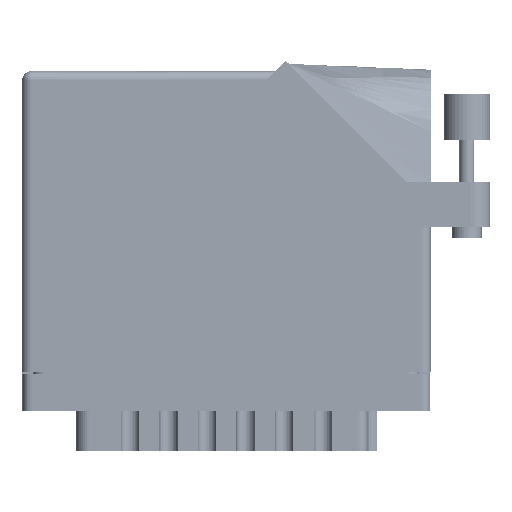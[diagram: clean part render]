
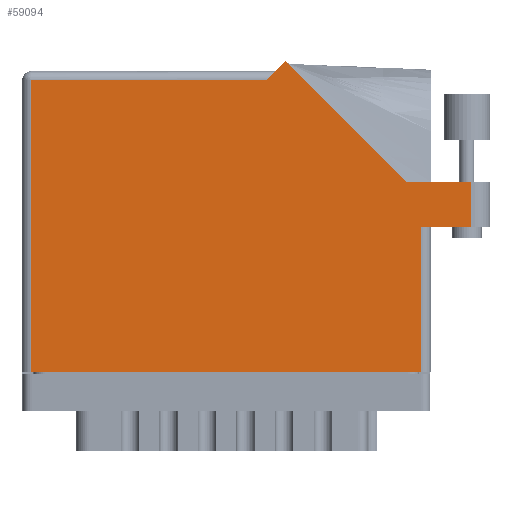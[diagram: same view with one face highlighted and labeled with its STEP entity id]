
A CAD part, front view. The second image highlights one B-rep face of the part: STEP entity #59094.
In plain terms, the highlighted face is planar.
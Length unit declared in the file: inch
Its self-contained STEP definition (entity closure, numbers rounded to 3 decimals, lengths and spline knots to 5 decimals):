
#2067 = ORIENTED_EDGE ( 'NONE', *, *, #8917, .T. ) ;
#4384 = LINE ( 'NONE', #84278, #96605 ) ;
#5635 = DIRECTION ( 'NONE',  ( 0., 0., -1. ) ) ;
#8917 = EDGE_CURVE ( 'NONE', #19180, #78501, #88058, .T. ) ;
#9292 = CARTESIAN_POINT ( 'NONE',  ( 0.062, 0., 0. ) ) ;
#9318 = DIRECTION ( 'NONE',  ( 0., 1., 0. ) ) ;
#10745 = CARTESIAN_POINT ( 'NONE',  ( 3.155, 1.287, 0. ) ) ;
#13589 = CARTESIAN_POINT ( 'NONE',  ( 1.643, 1.968, 0. ) ) ;
#14631 = EDGE_CURVE ( 'NONE', #51018, #41355, #78565, .T. ) ;
#19180 = VERTEX_POINT ( 'NONE', #47078 ) ;
#20090 = ORIENTED_EDGE ( 'NONE', *, *, #83629, .T. ) ;
#20225 = DIRECTION ( 'NONE',  ( -0.707, 0.707, 0. ) ) ;
#20840 = CARTESIAN_POINT ( 'NONE',  ( 2.58942, 1.287, 0. ) ) ;
#21300 = DIRECTION ( 'NONE',  ( -1., 0., 0. ) ) ;
#23514 = VECTOR ( 'NONE', #9318, 39.37008 ) ;
#31052 = EDGE_LOOP ( 'NONE', ( #64737, #20090, #2067, #32978, #32845, #91973, #91093, #93390, #40410 ) ) ;
#31656 = VERTEX_POINT ( 'NONE', #75558 ) ;
#32352 = VECTOR ( 'NONE', #45770, 39.37008 ) ;
#32845 = ORIENTED_EDGE ( 'NONE', *, *, #62433, .T. ) ;
#32978 = ORIENTED_EDGE ( 'NONE', *, *, #67503, .T. ) ;
#32984 = CARTESIAN_POINT ( 'NONE',  ( 1.77571, 2.10071, 0. ) ) ;
#33135 = VECTOR ( 'NONE', #64858, 39.37008 ) ;
#34730 = CARTESIAN_POINT ( 'NONE',  ( 0., 0., 0. ) ) ;
#35352 = CARTESIAN_POINT ( 'NONE',  ( 0., 2.03, 0. ) ) ;
#39279 = DIRECTION ( 'NONE',  ( -0.707, -0.707, 0. ) ) ;
#40410 = ORIENTED_EDGE ( 'NONE', *, *, #59574, .T. ) ;
#41355 = VERTEX_POINT ( 'NONE', #47971 ) ;
#43520 = VECTOR ( 'NONE', #91807, 39.37008 ) ;
#44281 = CARTESIAN_POINT ( 'NONE',  ( 0.062, 1.968, 0. ) ) ;
#45455 = LINE ( 'NONE', #20840, #48969 ) ;
#45770 = DIRECTION ( 'NONE',  ( 1., 0., 0. ) ) ;
#47078 = CARTESIAN_POINT ( 'NONE',  ( 3.03, 1.287, 0. ) ) ;
#47971 = CARTESIAN_POINT ( 'NONE',  ( 0.062, 0., 0. ) ) ;
#48245 = VECTOR ( 'NONE', #50005, 39.37008 ) ;
#48247 = CARTESIAN_POINT ( 'NONE',  ( 2.58942, 1.287, 0. ) ) ;
#48723 = CARTESIAN_POINT ( 'NONE',  ( 2.693, 0.98, 0. ) ) ;
#48969 = VECTOR ( 'NONE', #20225, 39.37008 ) ;
#50005 = DIRECTION ( 'NONE',  ( 1., 0., 0. ) ) ;
#50387 = EDGE_CURVE ( 'NONE', #89313, #53853, #61485, .T. ) ;
#51018 = VERTEX_POINT ( 'NONE', #44281 ) ;
#51528 = VERTEX_POINT ( 'NONE', #13589 ) ;
#52695 = LINE ( 'NONE', #76475, #23514 ) ;
#53853 = VERTEX_POINT ( 'NONE', #80790 ) ;
#55303 = LINE ( 'NONE', #94931, #33135 ) ;
#58978 = EDGE_CURVE ( 'NONE', #41355, #31656, #68061, .T. ) ;
#59094 = ADVANCED_FACE ( 'NONE', ( #93876 ), #73760, .F. ) ;
#59574 = EDGE_CURVE ( 'NONE', #31656, #89313, #55303, .T. ) ;
#60431 = CARTESIAN_POINT ( 'NONE',  ( 2.755, 0.98, 0. ) ) ;
#61485 = LINE ( 'NONE', #60431, #32352 ) ;
#62372 = VECTOR ( 'NONE', #62878, 39.37008 ) ;
#62433 = EDGE_CURVE ( 'NONE', #88732, #51528, #4384, .T. ) ;
#62878 = DIRECTION ( 'NONE',  ( -1., 0., 0. ) ) ;
#64737 = ORIENTED_EDGE ( 'NONE', *, *, #50387, .T. ) ;
#64858 = DIRECTION ( 'NONE',  ( 0., 1., 0. ) ) ;
#67503 = EDGE_CURVE ( 'NONE', #78501, #88732, #45455, .T. ) ;
#68061 = LINE ( 'NONE', #34730, #48245 ) ;
#71336 = DIRECTION ( 'NONE',  ( -1., 0., 0. ) ) ;
#72101 = VECTOR ( 'NONE', #71336, 39.37008 ) ;
#73760 = PLANE ( 'NONE',  #92888 ) ;
#75558 = CARTESIAN_POINT ( 'NONE',  ( 2.693, 0., 0. ) ) ;
#76475 = CARTESIAN_POINT ( 'NONE',  ( 3.03, 1.287, 0. ) ) ;
#78501 = VERTEX_POINT ( 'NONE', #48247 ) ;
#78565 = LINE ( 'NONE', #9292, #43520 ) ;
#80790 = CARTESIAN_POINT ( 'NONE',  ( 3.03, 0.98, 0. ) ) ;
#83629 = EDGE_CURVE ( 'NONE', #53853, #19180, #52695, .T. ) ;
#84278 = CARTESIAN_POINT ( 'NONE',  ( 1.705, 2.03, 0. ) ) ;
#84921 = LINE ( 'NONE', #94869, #72101 ) ;
#86389 = EDGE_CURVE ( 'NONE', #51528, #51018, #84921, .T. ) ;
#88058 = LINE ( 'NONE', #10745, #62372 ) ;
#88732 = VERTEX_POINT ( 'NONE', #32984 ) ;
#89313 = VERTEX_POINT ( 'NONE', #48723 ) ;
#91093 = ORIENTED_EDGE ( 'NONE', *, *, #14631, .T. ) ;
#91807 = DIRECTION ( 'NONE',  ( 0., -1., 0. ) ) ;
#91973 = ORIENTED_EDGE ( 'NONE', *, *, #86389, .T. ) ;
#92888 = AXIS2_PLACEMENT_3D ( 'NONE', #35352, #5635, #21300 ) ;
#93390 = ORIENTED_EDGE ( 'NONE', *, *, #58978, .T. ) ;
#93876 = FACE_OUTER_BOUND ( 'NONE', #31052, .T. ) ;
#94869 = CARTESIAN_POINT ( 'NONE',  ( 0., 1.968, 0. ) ) ;
#94931 = CARTESIAN_POINT ( 'NONE',  ( 2.693, 0.98, 0. ) ) ;
#96605 = VECTOR ( 'NONE', #39279, 39.37008 ) ;
